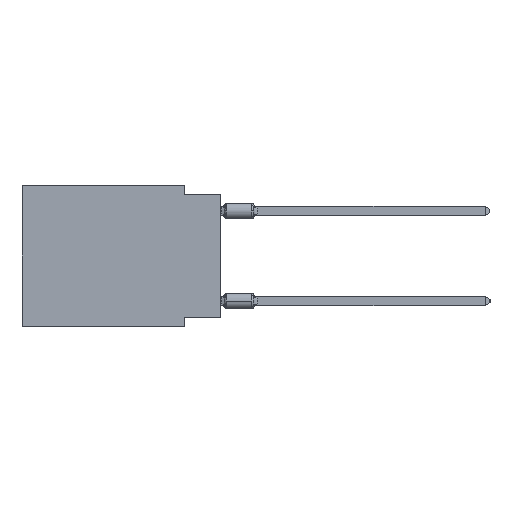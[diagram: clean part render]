
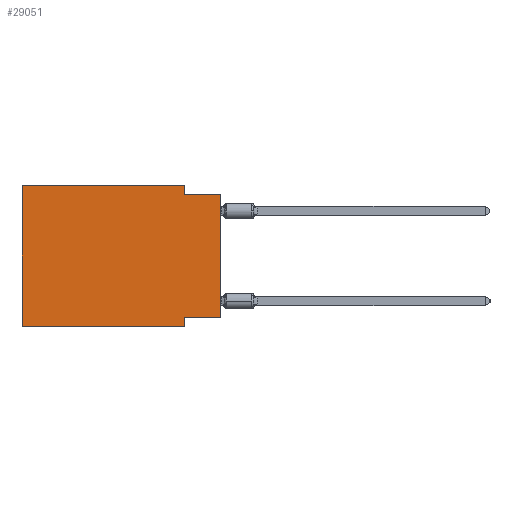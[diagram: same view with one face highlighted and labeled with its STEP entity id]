
A CAD part, left-side view. The second image highlights one B-rep face of the part: STEP entity #29051.
In plain terms, the highlighted planar face has unit normal (-1, 0, 0).
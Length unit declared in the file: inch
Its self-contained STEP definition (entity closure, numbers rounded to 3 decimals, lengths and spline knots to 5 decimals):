
#526 = VECTOR ( 'NONE', #1033, 39.37008 ) ;
#607 = DIRECTION ( 'NONE',  ( 1., 0., 0. ) ) ;
#1033 = DIRECTION ( 'NONE',  ( 0., 0., 1. ) ) ;
#2548 = CARTESIAN_POINT ( 'NONE',  ( 0., 0.1, -0.39 ) ) ;
#2785 = VECTOR ( 'NONE', #3996, 39.37008 ) ;
#3151 = VERTEX_POINT ( 'NONE', #26878 ) ;
#3589 = AXIS2_PLACEMENT_3D ( 'NONE', #20310, #607, #14097 ) ;
#3887 = EDGE_CURVE ( 'NONE', #23529, #3151, #15690, .T. ) ;
#3996 = DIRECTION ( 'NONE',  ( 0., 1., 0. ) ) ;
#4033 = CARTESIAN_POINT ( 'NONE',  ( 0., 0.1, -0.365 ) ) ;
#5161 = VECTOR ( 'NONE', #9078, 39.37008 ) ;
#5190 = ORIENTED_EDGE ( 'NONE', *, *, #11690, .T. ) ;
#5390 = VERTEX_POINT ( 'NONE', #34946 ) ;
#5849 = LINE ( 'NONE', #34579, #39280 ) ;
#6545 = ORIENTED_EDGE ( 'NONE', *, *, #10535, .F. ) ;
#6615 = CARTESIAN_POINT ( 'NONE',  ( 0., 0., -0.025 ) ) ;
#6847 = VERTEX_POINT ( 'NONE', #6615 ) ;
#7537 = CARTESIAN_POINT ( 'NONE',  ( 0., 0., -0.365 ) ) ;
#8188 = LINE ( 'NONE', #7537, #2785 ) ;
#8964 = EDGE_LOOP ( 'NONE', ( #5190, #34332, #6545, #23133, #29530, #23544, #33874, #29297 ) ) ;
#9078 = DIRECTION ( 'NONE',  ( 0., -1., 0. ) ) ;
#9960 = EDGE_CURVE ( 'NONE', #5390, #23529, #14935, .T. ) ;
#10535 = EDGE_CURVE ( 'NONE', #3151, #42133, #32413, .T. ) ;
#11273 = CARTESIAN_POINT ( 'NONE',  ( 0., 0.55, 0. ) ) ;
#11690 = EDGE_CURVE ( 'NONE', #21630, #6847, #41789, .T. ) ;
#12067 = VERTEX_POINT ( 'NONE', #4033 ) ;
#12919 = CARTESIAN_POINT ( 'NONE',  ( 0., 0.55, -0.39 ) ) ;
#13664 = EDGE_CURVE ( 'NONE', #21630, #12067, #8188, .T. ) ;
#13832 = EDGE_CURVE ( 'NONE', #42133, #6847, #28983, .T. ) ;
#14097 = DIRECTION ( 'NONE',  ( 0., 0., -1. ) ) ;
#14935 = LINE ( 'NONE', #28445, #23567 ) ;
#15690 = LINE ( 'NONE', #32986, #5161 ) ;
#18371 = CARTESIAN_POINT ( 'NONE',  ( 0., 0., -0.025 ) ) ;
#18658 = CARTESIAN_POINT ( 'NONE',  ( 0., 0., -0.365 ) ) ;
#18917 = LINE ( 'NONE', #12919, #20788 ) ;
#19327 = DIRECTION ( 'NONE',  ( 0., 0., -1. ) ) ;
#19354 = DIRECTION ( 'NONE',  ( 0., -1., 0. ) ) ;
#19865 = PLANE ( 'NONE',  #3589 ) ;
#20310 = CARTESIAN_POINT ( 'NONE',  ( 0., 0.55, 0. ) ) ;
#20788 = VECTOR ( 'NONE', #19354, 39.37008 ) ;
#21630 = VERTEX_POINT ( 'NONE', #18658 ) ;
#22574 = VECTOR ( 'NONE', #19327, 39.37008 ) ;
#23133 = ORIENTED_EDGE ( 'NONE', *, *, #3887, .F. ) ;
#23529 = VERTEX_POINT ( 'NONE', #11273 ) ;
#23544 = ORIENTED_EDGE ( 'NONE', *, *, #34936, .T. ) ;
#23567 = VECTOR ( 'NONE', #28893, 39.37008 ) ;
#24293 = FACE_OUTER_BOUND ( 'NONE', #8964, .T. ) ;
#25450 = DIRECTION ( 'NONE',  ( 0., -1., 0. ) ) ;
#26412 = CARTESIAN_POINT ( 'NONE',  ( 0., 0.1, 0. ) ) ;
#26878 = CARTESIAN_POINT ( 'NONE',  ( 0., 0.1, 0. ) ) ;
#27399 = CARTESIAN_POINT ( 'NONE',  ( 0., 0., 0. ) ) ;
#27688 = DIRECTION ( 'NONE',  ( 0., 0., -1. ) ) ;
#28445 = CARTESIAN_POINT ( 'NONE',  ( 0., 0.55, 0. ) ) ;
#28893 = DIRECTION ( 'NONE',  ( 0., 0., 1. ) ) ;
#28983 = LINE ( 'NONE', #18371, #39706 ) ;
#29051 = ADVANCED_FACE ( 'NONE', ( #24293 ), #19865, .F. ) ;
#29297 = ORIENTED_EDGE ( 'NONE', *, *, #13664, .F. ) ;
#29530 = ORIENTED_EDGE ( 'NONE', *, *, #9960, .F. ) ;
#32413 = LINE ( 'NONE', #26412, #22574 ) ;
#32986 = CARTESIAN_POINT ( 'NONE',  ( 0., 0.55, 0. ) ) ;
#33874 = ORIENTED_EDGE ( 'NONE', *, *, #36862, .F. ) ;
#34332 = ORIENTED_EDGE ( 'NONE', *, *, #13832, .F. ) ;
#34579 = CARTESIAN_POINT ( 'NONE',  ( 0., 0.1, -0.39 ) ) ;
#34936 = EDGE_CURVE ( 'NONE', #5390, #36834, #18917, .T. ) ;
#34946 = CARTESIAN_POINT ( 'NONE',  ( 0., 0.55, -0.39 ) ) ;
#36353 = CARTESIAN_POINT ( 'NONE',  ( 0., 0.1, -0.025 ) ) ;
#36834 = VERTEX_POINT ( 'NONE', #2548 ) ;
#36862 = EDGE_CURVE ( 'NONE', #12067, #36834, #5849, .T. ) ;
#39280 = VECTOR ( 'NONE', #27688, 39.37008 ) ;
#39706 = VECTOR ( 'NONE', #25450, 39.37008 ) ;
#41789 = LINE ( 'NONE', #27399, #526 ) ;
#42133 = VERTEX_POINT ( 'NONE', #36353 ) ;
